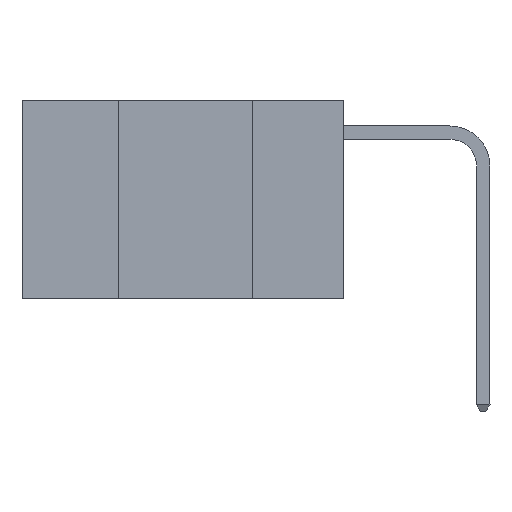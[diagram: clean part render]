
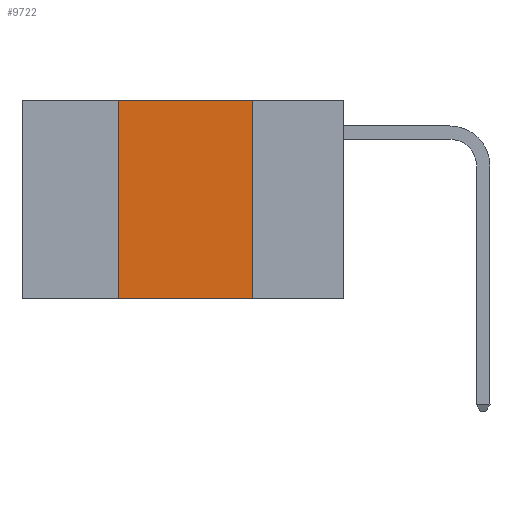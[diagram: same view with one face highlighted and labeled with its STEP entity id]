
A CAD part, left-side view. The second image highlights one B-rep face of the part: STEP entity #9722.
In plain terms, the highlighted planar face has unit normal (-1, 0, 0).
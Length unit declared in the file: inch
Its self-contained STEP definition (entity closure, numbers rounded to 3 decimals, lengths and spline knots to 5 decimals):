
#76 = CARTESIAN_POINT ( 'NONE',  ( 0., 0.42, 0. ) ) ;
#150 = DIRECTION ( 'NONE',  ( 0., 0., 1. ) ) ;
#852 = DIRECTION ( 'NONE',  ( 0., 0., -1. ) ) ;
#984 = CARTESIAN_POINT ( 'NONE',  ( 0., 0.42, 0. ) ) ;
#1312 = EDGE_LOOP ( 'NONE', ( #3670, #7975, #4173, #12737 ) ) ;
#1605 = VERTEX_POINT ( 'NONE', #15714 ) ;
#1798 = LINE ( 'NONE', #76, #14142 ) ;
#2238 = VERTEX_POINT ( 'NONE', #984 ) ;
#2421 = CARTESIAN_POINT ( 'NONE',  ( 0., 0.6, 0. ) ) ;
#2615 = AXIS2_PLACEMENT_3D ( 'NONE', #2421, #10589, #852 ) ;
#3209 = CARTESIAN_POINT ( 'NONE',  ( 0., 0.6, 0. ) ) ;
#3670 = ORIENTED_EDGE ( 'NONE', *, *, #15019, .F. ) ;
#4173 = ORIENTED_EDGE ( 'NONE', *, *, #11862, .F. ) ;
#5511 = DIRECTION ( 'NONE',  ( 0., 0., -1. ) ) ;
#5948 = VERTEX_POINT ( 'NONE', #17586 ) ;
#7120 = CARTESIAN_POINT ( 'NONE',  ( 0., 0.17, 0. ) ) ;
#7687 = LINE ( 'NONE', #3209, #19293 ) ;
#7975 = ORIENTED_EDGE ( 'NONE', *, *, #9527, .F. ) ;
#8653 = EDGE_CURVE ( 'NONE', #10517, #5948, #10031, .T. ) ;
#9308 = DIRECTION ( 'NONE',  ( 0., -1., 0. ) ) ;
#9455 = CARTESIAN_POINT ( 'NONE',  ( 0., 0.42, -0.37 ) ) ;
#9527 = EDGE_CURVE ( 'NONE', #2238, #1605, #7687, .T. ) ;
#9722 = ADVANCED_FACE ( 'NONE', ( #11695 ), #19951, .F. ) ;
#10031 = LINE ( 'NONE', #18701, #10521 ) ;
#10517 = VERTEX_POINT ( 'NONE', #9455 ) ;
#10521 = VECTOR ( 'NONE', #9308, 39.37008 ) ;
#10589 = DIRECTION ( 'NONE',  ( 1., 0., 0. ) ) ;
#11286 = DIRECTION ( 'NONE',  ( 0., -1., 0. ) ) ;
#11695 = FACE_OUTER_BOUND ( 'NONE', #1312, .T. ) ;
#11862 = EDGE_CURVE ( 'NONE', #10517, #2238, #1798, .T. ) ;
#12737 = ORIENTED_EDGE ( 'NONE', *, *, #8653, .T. ) ;
#14142 = VECTOR ( 'NONE', #150, 39.37008 ) ;
#14502 = VECTOR ( 'NONE', #5511, 39.37008 ) ;
#15019 = EDGE_CURVE ( 'NONE', #1605, #5948, #18659, .T. ) ;
#15714 = CARTESIAN_POINT ( 'NONE',  ( 0., 0.17, 0. ) ) ;
#17586 = CARTESIAN_POINT ( 'NONE',  ( 0., 0.17, -0.37 ) ) ;
#18659 = LINE ( 'NONE', #7120, #14502 ) ;
#18701 = CARTESIAN_POINT ( 'NONE',  ( 0., 0.6, -0.37 ) ) ;
#19293 = VECTOR ( 'NONE', #11286, 39.37008 ) ;
#19951 = PLANE ( 'NONE',  #2615 ) ;
